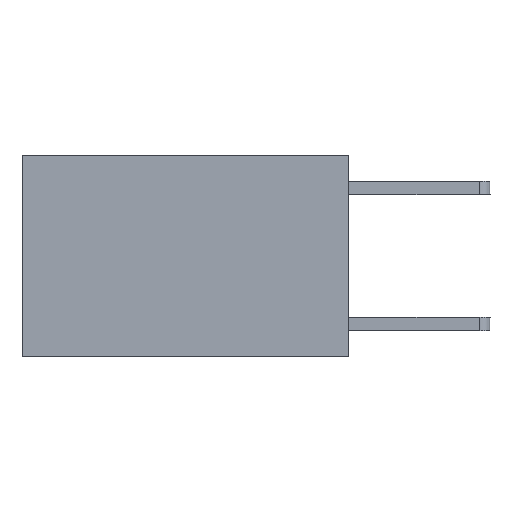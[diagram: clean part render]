
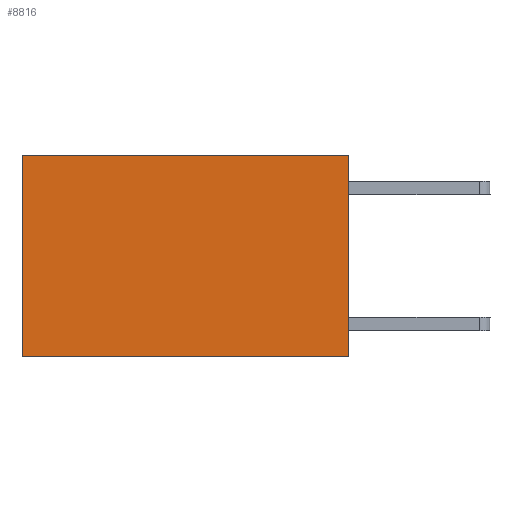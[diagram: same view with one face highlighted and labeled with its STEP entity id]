
A CAD part, left-side view. The second image highlights one B-rep face of the part: STEP entity #8816.
In plain terms, the highlighted planar face has unit normal (-1, 0, 0).
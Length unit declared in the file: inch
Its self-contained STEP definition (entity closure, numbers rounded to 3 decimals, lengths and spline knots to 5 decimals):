
#115 = VECTOR ( 'NONE', #4720, 39.37008 ) ;
#143 = EDGE_CURVE ( 'NONE', #2448, #6013, #1961, .T. ) ;
#347 = VECTOR ( 'NONE', #7240, 39.37008 ) ;
#403 = EDGE_CURVE ( 'NONE', #1553, #6013, #6975, .T. ) ;
#458 = CARTESIAN_POINT ( 'NONE',  ( 0.2625, 0., -0.37 ) ) ;
#911 = CARTESIAN_POINT ( 'NONE',  ( 0.2625, 0.6, 0. ) ) ;
#956 = DIRECTION ( 'NONE',  ( 0., 1., 0. ) ) ;
#1449 = EDGE_LOOP ( 'NONE', ( #2204, #4566, #9099, #6890 ) ) ;
#1553 = VERTEX_POINT ( 'NONE', #4069 ) ;
#1649 = CARTESIAN_POINT ( 'NONE',  ( 0.2625, 0.6, -0.37 ) ) ;
#1961 = LINE ( 'NONE', #458, #347 ) ;
#2204 = ORIENTED_EDGE ( 'NONE', *, *, #403, .T. ) ;
#2268 = VERTEX_POINT ( 'NONE', #3988 ) ;
#2448 = VERTEX_POINT ( 'NONE', #3523 ) ;
#2820 = DIRECTION ( 'NONE',  ( 1., 0., 0. ) ) ;
#3142 = AXIS2_PLACEMENT_3D ( 'NONE', #9736, #2820, #5899 ) ;
#3469 = VECTOR ( 'NONE', #8341, 39.37008 ) ;
#3523 = CARTESIAN_POINT ( 'NONE',  ( 0.2625, 0., -0.37 ) ) ;
#3988 = CARTESIAN_POINT ( 'NONE',  ( 0.2625, 0., 0. ) ) ;
#4069 = CARTESIAN_POINT ( 'NONE',  ( 0.2625, 0.6, 0. ) ) ;
#4566 = ORIENTED_EDGE ( 'NONE', *, *, #143, .F. ) ;
#4720 = DIRECTION ( 'NONE',  ( 0., 0., -1. ) ) ;
#5257 = CARTESIAN_POINT ( 'NONE',  ( 0.2625, 0., 0. ) ) ;
#5340 = EDGE_CURVE ( 'NONE', #2268, #2448, #9155, .T. ) ;
#5899 = DIRECTION ( 'NONE',  ( 0., 0., -1. ) ) ;
#6013 = VERTEX_POINT ( 'NONE', #1649 ) ;
#6262 = CARTESIAN_POINT ( 'NONE',  ( 0.2625, 0., 0. ) ) ;
#6786 = LINE ( 'NONE', #6262, #7334 ) ;
#6865 = PLANE ( 'NONE',  #3142 ) ;
#6890 = ORIENTED_EDGE ( 'NONE', *, *, #7232, .T. ) ;
#6975 = LINE ( 'NONE', #911, #115 ) ;
#7232 = EDGE_CURVE ( 'NONE', #2268, #1553, #6786, .T. ) ;
#7240 = DIRECTION ( 'NONE',  ( 0., 1., 0. ) ) ;
#7334 = VECTOR ( 'NONE', #956, 39.37008 ) ;
#8341 = DIRECTION ( 'NONE',  ( 0., 0., -1. ) ) ;
#8379 = FACE_OUTER_BOUND ( 'NONE', #1449, .T. ) ;
#8816 = ADVANCED_FACE ( 'NONE', ( #8379 ), #6865, .F. ) ;
#9099 = ORIENTED_EDGE ( 'NONE', *, *, #5340, .F. ) ;
#9155 = LINE ( 'NONE', #5257, #3469 ) ;
#9736 = CARTESIAN_POINT ( 'NONE',  ( 0.2625, 0., 0. ) ) ;
